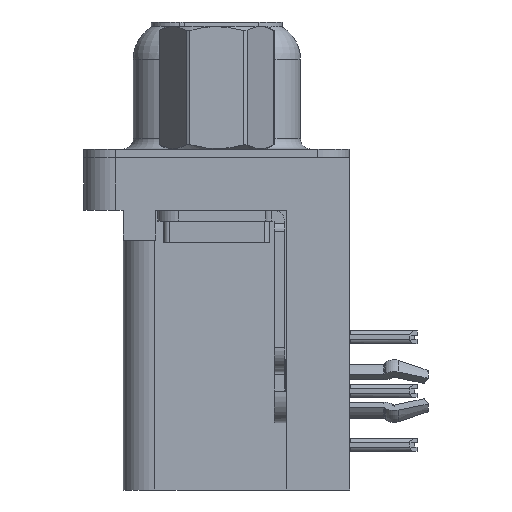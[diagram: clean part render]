
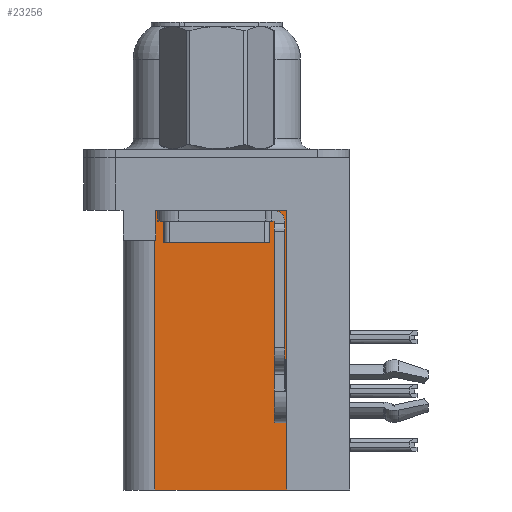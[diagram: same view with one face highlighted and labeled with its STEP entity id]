
A CAD part, left-side view. The second image highlights one B-rep face of the part: STEP entity #23256.
In plain terms, the highlighted planar face has unit normal (-1, 0, 0).
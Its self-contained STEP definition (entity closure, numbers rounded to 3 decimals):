
#754 = DIRECTION ( 'NONE',  ( 0., 0., -1. ) ) ;
#1092 = DIRECTION ( 'NONE',  ( 0., 0., -1. ) ) ;
#1432 = VERTEX_POINT ( 'NONE', #38623 ) ;
#1490 = CARTESIAN_POINT ( 'NONE',  ( 3.765, 2.925, -15.7 ) ) ;
#1618 = CARTESIAN_POINT ( 'NONE',  ( 3.765, 2.925, -3.9 ) ) ;
#1709 = FACE_OUTER_BOUND ( 'NONE', #2857, .T. ) ;
#2459 = EDGE_CURVE ( 'NONE', #12673, #1432, #15141, .T. ) ;
#2857 = EDGE_LOOP ( 'NONE', ( #11468, #7657, #31897, #39189, #3804, #13452 ) ) ;
#3660 = CARTESIAN_POINT ( 'NONE',  ( 3.765, -3.295, -15.7 ) ) ;
#3804 = ORIENTED_EDGE ( 'NONE', *, *, #29153, .F. ) ;
#3979 = LINE ( 'NONE', #3660, #38504 ) ;
#5549 = VECTOR ( 'NONE', #754, 1000. ) ;
#5904 = EDGE_CURVE ( 'NONE', #1432, #9466, #26428, .T. ) ;
#6227 = VECTOR ( 'NONE', #6314, 1000. ) ;
#6314 = DIRECTION ( 'NONE',  ( 0., 1., 0. ) ) ;
#7657 = ORIENTED_EDGE ( 'NONE', *, *, #5904, .T. ) ;
#8415 = LINE ( 'NONE', #26455, #28295 ) ;
#9466 = VERTEX_POINT ( 'NONE', #28275 ) ;
#10165 = EDGE_CURVE ( 'NONE', #9466, #11614, #8415, .T. ) ;
#10985 = PLANE ( 'NONE',  #31996 ) ;
#11219 = VERTEX_POINT ( 'NONE', #15136 ) ;
#11468 = ORIENTED_EDGE ( 'NONE', *, *, #2459, .T. ) ;
#11614 = VERTEX_POINT ( 'NONE', #1618 ) ;
#12673 = VERTEX_POINT ( 'NONE', #36066 ) ;
#13452 = ORIENTED_EDGE ( 'NONE', *, *, #29421, .T. ) ;
#14411 = CARTESIAN_POINT ( 'NONE',  ( 3.765, -3.295, -15.7 ) ) ;
#15136 = CARTESIAN_POINT ( 'NONE',  ( 3.765, 2.925, -15.7 ) ) ;
#15141 = LINE ( 'NONE', #32593, #6227 ) ;
#15639 = DIRECTION ( 'NONE',  ( 0., 0., 1. ) ) ;
#19744 = DIRECTION ( 'NONE',  ( 0., 1., 0. ) ) ;
#21060 = DIRECTION ( 'NONE',  ( 1., 0., 0. ) ) ;
#21170 = LINE ( 'NONE', #25514, #37948 ) ;
#21467 = DIRECTION ( 'NONE',  ( 0., 0., 1. ) ) ;
#22949 = VECTOR ( 'NONE', #21467, 1000. ) ;
#23256 = ADVANCED_FACE ( 'NONE', ( #1709 ), #10985, .F. ) ;
#23984 = LINE ( 'NONE', #1490, #22949 ) ;
#25514 = CARTESIAN_POINT ( 'NONE',  ( 3.765, -3.295, -15.7 ) ) ;
#26428 = LINE ( 'NONE', #37446, #5549 ) ;
#26455 = CARTESIAN_POINT ( 'NONE',  ( 3.765, 0., -3.9 ) ) ;
#26545 = EDGE_CURVE ( 'NONE', #11219, #11614, #23984, .T. ) ;
#28275 = CARTESIAN_POINT ( 'NONE',  ( 3.765, 2.895, -3.9 ) ) ;
#28295 = VECTOR ( 'NONE', #19744, 1000. ) ;
#29153 = EDGE_CURVE ( 'NONE', #32347, #11219, #3979, .T. ) ;
#29421 = EDGE_CURVE ( 'NONE', #32347, #12673, #21170, .T. ) ;
#30431 = DIRECTION ( 'NONE',  ( 0., 1., 0. ) ) ;
#31897 = ORIENTED_EDGE ( 'NONE', *, *, #10165, .T. ) ;
#31996 = AXIS2_PLACEMENT_3D ( 'NONE', #14411, #21060, #1092 ) ;
#32347 = VERTEX_POINT ( 'NONE', #35151 ) ;
#32593 = CARTESIAN_POINT ( 'NONE',  ( 3.765, -3.295, -2.5 ) ) ;
#35151 = CARTESIAN_POINT ( 'NONE',  ( 3.765, -3.295, -15.7 ) ) ;
#36066 = CARTESIAN_POINT ( 'NONE',  ( 3.765, -3.295, -2.5 ) ) ;
#37446 = CARTESIAN_POINT ( 'NONE',  ( 3.765, 2.895, -3.9 ) ) ;
#37948 = VECTOR ( 'NONE', #15639, 1000. ) ;
#38504 = VECTOR ( 'NONE', #30431, 1000. ) ;
#38623 = CARTESIAN_POINT ( 'NONE',  ( 3.765, 2.895, -2.5 ) ) ;
#39189 = ORIENTED_EDGE ( 'NONE', *, *, #26545, .F. ) ;
